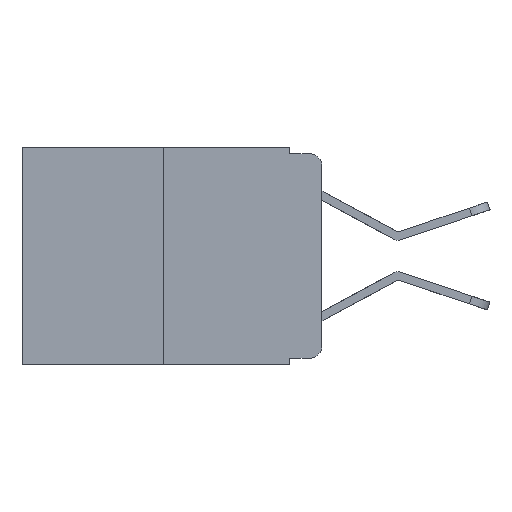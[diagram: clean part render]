
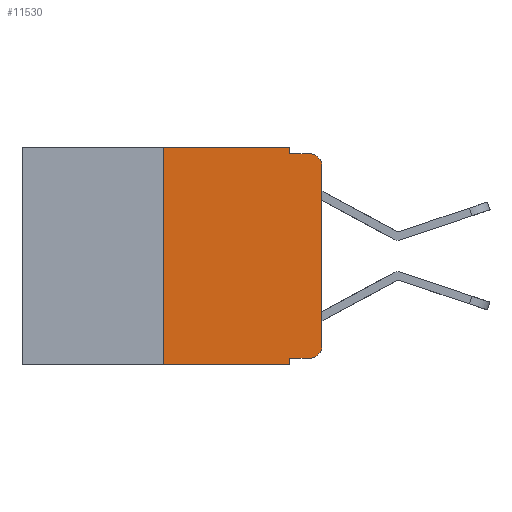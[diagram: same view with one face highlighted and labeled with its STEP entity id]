
A CAD part, left-side view. The second image highlights one B-rep face of the part: STEP entity #11530.
In plain terms, the highlighted planar face has unit normal (-1, 0, 0).
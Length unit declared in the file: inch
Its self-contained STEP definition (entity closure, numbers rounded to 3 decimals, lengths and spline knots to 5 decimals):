
#600 = VECTOR ( 'NONE', #9269, 39.37008 ) ;
#952 = CARTESIAN_POINT ( 'NONE',  ( 0., 0.02, -0.01 ) ) ;
#1505 = VECTOR ( 'NONE', #8767, 39.37008 ) ;
#2381 = DIRECTION ( 'NONE',  ( 0., 0., 1. ) ) ;
#2506 = CARTESIAN_POINT ( 'NONE',  ( 0., 0.473, -0.343 ) ) ;
#2983 = VERTEX_POINT ( 'NONE', #6191 ) ;
#3581 = ORIENTED_EDGE ( 'NONE', *, *, #18643, .T. ) ;
#3602 = CARTESIAN_POINT ( 'NONE',  ( 0., 0.473, 0. ) ) ;
#4146 = ORIENTED_EDGE ( 'NONE', *, *, #16627, .F. ) ;
#4803 = CARTESIAN_POINT ( 'NONE',  ( 0., 0., -0.03 ) ) ;
#5738 = ORIENTED_EDGE ( 'NONE', *, *, #12633, .T. ) ;
#5894 = CARTESIAN_POINT ( 'NONE',  ( 0., 0.25, 0. ) ) ;
#6179 = LINE ( 'NONE', #3602, #1505 ) ;
#6191 = CARTESIAN_POINT ( 'NONE',  ( 0., 0.02, -0.333 ) ) ;
#6264 = VERTEX_POINT ( 'NONE', #18466 ) ;
#6590 = DIRECTION ( 'NONE',  ( -1., 0., 0. ) ) ;
#6772 = AXIS2_PLACEMENT_3D ( 'NONE', #12146, #8832, #20326 ) ;
#6874 = ORIENTED_EDGE ( 'NONE', *, *, #10886, .F. ) ;
#6993 = DIRECTION ( 'NONE',  ( 0., 0., -1. ) ) ;
#7000 = VECTOR ( 'NONE', #9628, 39.37008 ) ;
#7089 = CARTESIAN_POINT ( 'NONE',  ( 0., 0.051, 0. ) ) ;
#7317 = CARTESIAN_POINT ( 'NONE',  ( 0., 0.051, -0.01 ) ) ;
#7492 = ORIENTED_EDGE ( 'NONE', *, *, #19512, .F. ) ;
#7564 = ORIENTED_EDGE ( 'NONE', *, *, #7624, .T. ) ;
#7624 = EDGE_CURVE ( 'NONE', #18069, #2983, #20187, .T. ) ;
#7860 = ORIENTED_EDGE ( 'NONE', *, *, #18203, .F. ) ;
#8189 = ORIENTED_EDGE ( 'NONE', *, *, #11681, .T. ) ;
#8237 = EDGE_LOOP ( 'NONE', ( #5738, #3581, #4146, #10507, #7860, #7492, #8189, #6874, #7564, #14413 ) ) ;
#8292 = CIRCLE ( 'NONE', #9849, 0.02 ) ;
#8300 = DIRECTION ( 'NONE',  ( -1., 0., 0. ) ) ;
#8767 = DIRECTION ( 'NONE',  ( 0., -1., 0. ) ) ;
#8832 = DIRECTION ( 'NONE',  ( 1., 0., 0. ) ) ;
#9130 = VERTEX_POINT ( 'NONE', #21709 ) ;
#9269 = DIRECTION ( 'NONE',  ( 0., 0., -1. ) ) ;
#9628 = DIRECTION ( 'NONE',  ( 0., -1., 0. ) ) ;
#9849 = AXIS2_PLACEMENT_3D ( 'NONE', #16588, #6590, #18216 ) ;
#10090 = EDGE_CURVE ( 'NONE', #2983, #6264, #16997, .T. ) ;
#10289 = VERTEX_POINT ( 'NONE', #7089 ) ;
#10507 = ORIENTED_EDGE ( 'NONE', *, *, #18943, .F. ) ;
#10886 = EDGE_CURVE ( 'NONE', #18069, #12903, #15196, .T. ) ;
#11007 = VECTOR ( 'NONE', #11736, 39.37008 ) ;
#11132 = DIRECTION ( 'NONE',  ( 0., -1., 0. ) ) ;
#11259 = VECTOR ( 'NONE', #18898, 39.37008 ) ;
#11530 = ADVANCED_FACE ( 'NONE', ( #15936 ), #18723, .F. ) ;
#11681 = EDGE_CURVE ( 'NONE', #12112, #12903, #20973, .T. ) ;
#11685 = LINE ( 'NONE', #5894, #19848 ) ;
#11736 = DIRECTION ( 'NONE',  ( 0., 0., 1. ) ) ;
#12112 = VERTEX_POINT ( 'NONE', #20310 ) ;
#12140 = VERTEX_POINT ( 'NONE', #17207 ) ;
#12146 = CARTESIAN_POINT ( 'NONE',  ( 0., 0.473, 0. ) ) ;
#12633 = EDGE_CURVE ( 'NONE', #6264, #18648, #15393, .T. ) ;
#12903 = VERTEX_POINT ( 'NONE', #15752 ) ;
#13411 = CARTESIAN_POINT ( 'NONE',  ( 0., 0., 0. ) ) ;
#13789 = LINE ( 'NONE', #19118, #600 ) ;
#14170 = VECTOR ( 'NONE', #6993, 39.37008 ) ;
#14413 = ORIENTED_EDGE ( 'NONE', *, *, #10090, .T. ) ;
#15196 = LINE ( 'NONE', #16973, #14170 ) ;
#15393 = LINE ( 'NONE', #13411, #11007 ) ;
#15634 = LINE ( 'NONE', #7317, #11259 ) ;
#15752 = CARTESIAN_POINT ( 'NONE',  ( 0., 0.051, -0.343 ) ) ;
#15936 = FACE_OUTER_BOUND ( 'NONE', #8237, .T. ) ;
#16126 = CARTESIAN_POINT ( 'NONE',  ( 0., 0.051, -0.333 ) ) ;
#16588 = CARTESIAN_POINT ( 'NONE',  ( 0., 0.02, -0.03 ) ) ;
#16627 = EDGE_CURVE ( 'NONE', #12140, #20913, #15634, .T. ) ;
#16973 = CARTESIAN_POINT ( 'NONE',  ( 0., 0.051, 0. ) ) ;
#16997 = CIRCLE ( 'NONE', #20322, 0.02 ) ;
#17207 = CARTESIAN_POINT ( 'NONE',  ( 0., 0.051, -0.01 ) ) ;
#18069 = VERTEX_POINT ( 'NONE', #18073 ) ;
#18073 = CARTESIAN_POINT ( 'NONE',  ( 0., 0.051, -0.333 ) ) ;
#18203 = EDGE_CURVE ( 'NONE', #9130, #10289, #6179, .T. ) ;
#18214 = CARTESIAN_POINT ( 'NONE',  ( 0., 0.02, -0.313 ) ) ;
#18216 = DIRECTION ( 'NONE',  ( 0., 0., -1. ) ) ;
#18466 = CARTESIAN_POINT ( 'NONE',  ( 0., 0., -0.313 ) ) ;
#18643 = EDGE_CURVE ( 'NONE', #18648, #20913, #8292, .T. ) ;
#18648 = VERTEX_POINT ( 'NONE', #4803 ) ;
#18723 = PLANE ( 'NONE',  #6772 ) ;
#18898 = DIRECTION ( 'NONE',  ( 0., -1., 0. ) ) ;
#18943 = EDGE_CURVE ( 'NONE', #10289, #12140, #13789, .T. ) ;
#19118 = CARTESIAN_POINT ( 'NONE',  ( 0., 0.051, 0. ) ) ;
#19512 = EDGE_CURVE ( 'NONE', #12112, #9130, #11685, .T. ) ;
#19830 = DIRECTION ( 'NONE',  ( 0., 0., -1. ) ) ;
#19848 = VECTOR ( 'NONE', #2381, 39.37008 ) ;
#20187 = LINE ( 'NONE', #16126, #7000 ) ;
#20310 = CARTESIAN_POINT ( 'NONE',  ( 0., 0.25, -0.343 ) ) ;
#20322 = AXIS2_PLACEMENT_3D ( 'NONE', #18214, #8300, #19830 ) ;
#20326 = DIRECTION ( 'NONE',  ( 0., 0., -1. ) ) ;
#20913 = VERTEX_POINT ( 'NONE', #952 ) ;
#20973 = LINE ( 'NONE', #2506, #21478 ) ;
#21478 = VECTOR ( 'NONE', #11132, 39.37008 ) ;
#21709 = CARTESIAN_POINT ( 'NONE',  ( 0., 0.25, 0. ) ) ;
